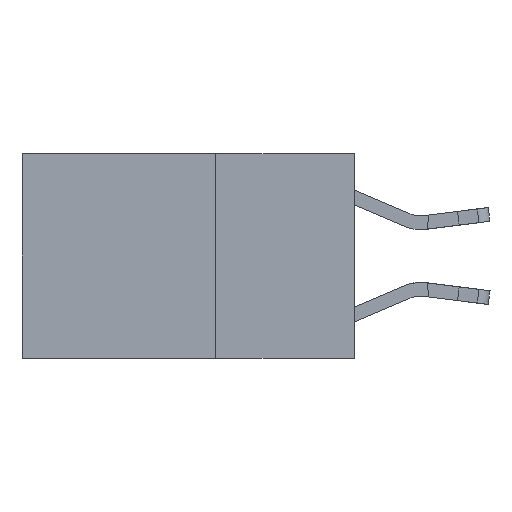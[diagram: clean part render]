
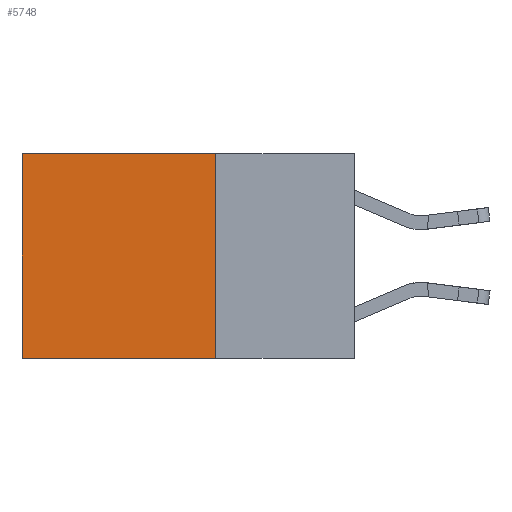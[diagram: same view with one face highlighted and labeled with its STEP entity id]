
A CAD part, left-side view. The second image highlights one B-rep face of the part: STEP entity #5748.
In plain terms, the highlighted planar face has unit normal (-1, 0, 0).
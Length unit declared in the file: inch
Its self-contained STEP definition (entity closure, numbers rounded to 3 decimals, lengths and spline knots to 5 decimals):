
#1349 = DIRECTION ( 'NONE',  ( 1., 0., 0. ) ) ;
#1637 = VECTOR ( 'NONE', #22500, 39.37008 ) ;
#2225 = VERTEX_POINT ( 'NONE', #10205 ) ;
#3063 = CARTESIAN_POINT ( 'NONE',  ( 0.2625, 0.25, 0. ) ) ;
#3778 = EDGE_CURVE ( 'NONE', #2225, #5330, #18937, .T. ) ;
#4175 = ORIENTED_EDGE ( 'NONE', *, *, #3778, .T. ) ;
#5330 = VERTEX_POINT ( 'NONE', #10807 ) ;
#5748 = ADVANCED_FACE ( 'NONE', ( #9254 ), #17507, .F. ) ;
#6735 = CARTESIAN_POINT ( 'NONE',  ( 0.2625, 0.25, -0.37 ) ) ;
#6997 = ORIENTED_EDGE ( 'NONE', *, *, #13640, .F. ) ;
#7921 = CARTESIAN_POINT ( 'NONE',  ( 0.2625, 0.6, 0. ) ) ;
#9254 = FACE_OUTER_BOUND ( 'NONE', #17893, .T. ) ;
#10205 = CARTESIAN_POINT ( 'NONE',  ( 0.2625, 0.25, 0. ) ) ;
#10333 = CARTESIAN_POINT ( 'NONE',  ( 0.2625, 0.6, -0.37 ) ) ;
#10379 = DIRECTION ( 'NONE',  ( 0., 0., -1. ) ) ;
#10527 = EDGE_CURVE ( 'NONE', #5330, #18075, #13345, .T. ) ;
#10807 = CARTESIAN_POINT ( 'NONE',  ( 0.2625, 0.6, 0. ) ) ;
#13345 = LINE ( 'NONE', #7921, #18002 ) ;
#13640 = EDGE_CURVE ( 'NONE', #2225, #19389, #19529, .T. ) ;
#14273 = VECTOR ( 'NONE', #22350, 39.37008 ) ;
#14885 = VECTOR ( 'NONE', #10379, 39.37008 ) ;
#15750 = CARTESIAN_POINT ( 'NONE',  ( 0.2625, 0.25, 0. ) ) ;
#17507 = PLANE ( 'NONE',  #21924 ) ;
#17893 = EDGE_LOOP ( 'NONE', ( #21506, #21610, #6997, #4175 ) ) ;
#18002 = VECTOR ( 'NONE', #18369, 39.37008 ) ;
#18075 = VERTEX_POINT ( 'NONE', #10333 ) ;
#18180 = CARTESIAN_POINT ( 'NONE',  ( 0.2625, 0.25, -0.37 ) ) ;
#18369 = DIRECTION ( 'NONE',  ( 0., 0., -1. ) ) ;
#18937 = LINE ( 'NONE', #20641, #14273 ) ;
#19284 = DIRECTION ( 'NONE',  ( 0., 0., -1. ) ) ;
#19389 = VERTEX_POINT ( 'NONE', #18180 ) ;
#19529 = LINE ( 'NONE', #3063, #14885 ) ;
#20641 = CARTESIAN_POINT ( 'NONE',  ( 0.2625, 0.25, 0. ) ) ;
#20651 = LINE ( 'NONE', #6735, #1637 ) ;
#20794 = EDGE_CURVE ( 'NONE', #19389, #18075, #20651, .T. ) ;
#21506 = ORIENTED_EDGE ( 'NONE', *, *, #10527, .T. ) ;
#21610 = ORIENTED_EDGE ( 'NONE', *, *, #20794, .F. ) ;
#21924 = AXIS2_PLACEMENT_3D ( 'NONE', #15750, #1349, #19284 ) ;
#22350 = DIRECTION ( 'NONE',  ( 0., 1., 0. ) ) ;
#22500 = DIRECTION ( 'NONE',  ( 0., 1., 0. ) ) ;
